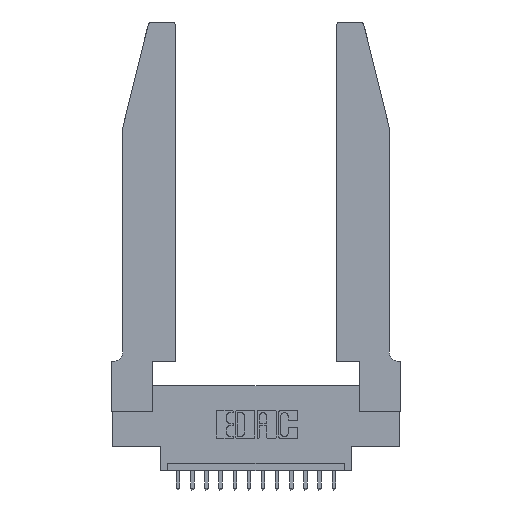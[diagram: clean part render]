
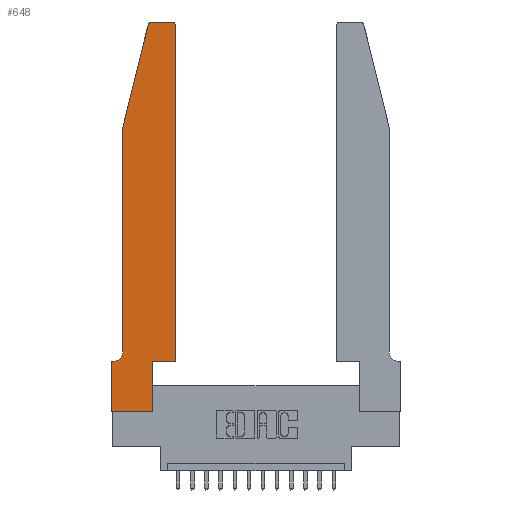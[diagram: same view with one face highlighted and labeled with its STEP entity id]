
A CAD part, top view. The second image highlights one B-rep face of the part: STEP entity #648.
In plain terms, the highlighted planar face has unit normal (0, 0, 1).
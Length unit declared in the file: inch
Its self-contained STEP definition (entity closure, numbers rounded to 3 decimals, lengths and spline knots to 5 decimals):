
#505 = VECTOR ( 'NONE', #3191, 39.37008 ) ;
#648 = ADVANCED_FACE ( 'NONE', ( #2375 ), #1194, .T. ) ;
#860 = CARTESIAN_POINT ( 'NONE',  ( 0.0055, 0.35, 0.37 ) ) ;
#938 = AXIS2_PLACEMENT_3D ( 'NONE', #9740, #6860, #15231 ) ;
#978 = ORIENTED_EDGE ( 'NONE', *, *, #1954, .T. ) ;
#1126 = CARTESIAN_POINT ( 'NONE',  ( 0.4205, 2.72, 0.37 ) ) ;
#1164 = DIRECTION ( 'NONE',  ( 1., 0., 0. ) ) ;
#1194 = PLANE ( 'NONE',  #938 ) ;
#1410 = CIRCLE ( 'NONE', #11759, 0.03 ) ;
#1486 = EDGE_LOOP ( 'NONE', ( #7012, #6989, #10136, #8516, #10337, #12868, #978, #15834, #2929, #10157, #9192, #16131 ) ) ;
#1492 = DIRECTION ( 'NONE',  ( -1., 0., 0. ) ) ;
#1592 = CIRCLE ( 'NONE', #3282, 0.03 ) ;
#1691 = VERTEX_POINT ( 'NONE', #3561 ) ;
#1754 = EDGE_CURVE ( 'NONE', #7570, #12493, #9913, .T. ) ;
#1954 = EDGE_CURVE ( 'NONE', #10175, #7570, #10794, .T. ) ;
#2098 = CARTESIAN_POINT ( 'NONE',  ( 0.2865, 0., 0.37 ) ) ;
#2114 = DIRECTION ( 'NONE',  ( 0., 0., -1. ) ) ;
#2375 = FACE_OUTER_BOUND ( 'NONE', #1486, .T. ) ;
#2431 = VERTEX_POINT ( 'NONE', #11007 ) ;
#2732 = CARTESIAN_POINT ( 'NONE',  ( 0.0755, 0.42, 0.37 ) ) ;
#2853 = CARTESIAN_POINT ( 'NONE',  ( 0.0755, 2., 0.37 ) ) ;
#2929 = ORIENTED_EDGE ( 'NONE', *, *, #4410, .T. ) ;
#3191 = DIRECTION ( 'NONE',  ( -0.239, -0.971, 0. ) ) ;
#3282 = AXIS2_PLACEMENT_3D ( 'NONE', #17812, #9458, #1164 ) ;
#3397 = VECTOR ( 'NONE', #14045, 39.37008 ) ;
#3463 = EDGE_CURVE ( 'NONE', #2431, #10701, #1592, .T. ) ;
#3561 = CARTESIAN_POINT ( 'NONE',  ( 0.4505, 2.72, 0.37 ) ) ;
#3717 = VERTEX_POINT ( 'NONE', #860 ) ;
#3766 = AXIS2_PLACEMENT_3D ( 'NONE', #13324, #2114, #9040 ) ;
#4410 = EDGE_CURVE ( 'NONE', #12493, #5155, #17122, .T. ) ;
#4894 = EDGE_CURVE ( 'NONE', #3717, #10175, #13527, .T. ) ;
#5096 = VECTOR ( 'NONE', #10416, 39.37008 ) ;
#5155 = VERTEX_POINT ( 'NONE', #15409 ) ;
#5196 = EDGE_CURVE ( 'NONE', #10701, #12759, #17670, .T. ) ;
#5198 = VERTEX_POINT ( 'NONE', #5371 ) ;
#5371 = CARTESIAN_POINT ( 'NONE',  ( 0.4505, 0.35, 0.37 ) ) ;
#5412 = CARTESIAN_POINT ( 'NONE',  ( 0.0755, 2., 0.37 ) ) ;
#5843 = CARTESIAN_POINT ( 'NONE',  ( 0.2865, 0.35, 0.37 ) ) ;
#6199 = VECTOR ( 'NONE', #14973, 39.37008 ) ;
#6245 = VECTOR ( 'NONE', #17843, 39.37008 ) ;
#6577 = DIRECTION ( 'NONE',  ( 0., 1., 0. ) ) ;
#6606 = DIRECTION ( 'NONE',  ( 1., 0., 0. ) ) ;
#6827 = EDGE_CURVE ( 'NONE', #5155, #5198, #16113, .T. ) ;
#6860 = DIRECTION ( 'NONE',  ( 0., 0., 1. ) ) ;
#6955 = VECTOR ( 'NONE', #7656, 39.37008 ) ;
#6989 = ORIENTED_EDGE ( 'NONE', *, *, #3463, .T. ) ;
#7012 = ORIENTED_EDGE ( 'NONE', *, *, #11635, .T. ) ;
#7280 = EDGE_CURVE ( 'NONE', #11071, #3717, #8637, .T. ) ;
#7570 = VERTEX_POINT ( 'NONE', #12748 ) ;
#7656 = DIRECTION ( 'NONE',  ( 1., 0., 0. ) ) ;
#8516 = ORIENTED_EDGE ( 'NONE', *, *, #12175, .T. ) ;
#8607 = CARTESIAN_POINT ( 'NONE',  ( 0.4505, 0.35, 0.37 ) ) ;
#8637 = CIRCLE ( 'NONE', #3766, 0.07 ) ;
#8858 = VERTEX_POINT ( 'NONE', #16887 ) ;
#8970 = CARTESIAN_POINT ( 'NONE',  ( 0.4505, 0.35, 0.37 ) ) ;
#9040 = DIRECTION ( 'NONE',  ( -1., 0., 0. ) ) ;
#9192 = ORIENTED_EDGE ( 'NONE', *, *, #15485, .T. ) ;
#9458 = DIRECTION ( 'NONE',  ( 0., 0., 1. ) ) ;
#9634 = LINE ( 'NONE', #2853, #5096 ) ;
#9671 = CARTESIAN_POINT ( 'NONE',  ( 0.0755, 2., 0.37 ) ) ;
#9740 = CARTESIAN_POINT ( 'NONE',  ( 0., 0.35, 0.37 ) ) ;
#9844 = VECTOR ( 'NONE', #1492, 39.37008 ) ;
#9913 = LINE ( 'NONE', #15040, #6245 ) ;
#10136 = ORIENTED_EDGE ( 'NONE', *, *, #5196, .T. ) ;
#10157 = ORIENTED_EDGE ( 'NONE', *, *, #6827, .T. ) ;
#10166 = LINE ( 'NONE', #8607, #15393 ) ;
#10175 = VERTEX_POINT ( 'NONE', #14921 ) ;
#10337 = ORIENTED_EDGE ( 'NONE', *, *, #7280, .T. ) ;
#10416 = DIRECTION ( 'NONE',  ( 0., -1., 0. ) ) ;
#10701 = VERTEX_POINT ( 'NONE', #11785 ) ;
#10794 = LINE ( 'NONE', #16627, #3397 ) ;
#11007 = CARTESIAN_POINT ( 'NONE',  ( 0.284, 2.75, 0.37 ) ) ;
#11071 = VERTEX_POINT ( 'NONE', #2732 ) ;
#11384 = VECTOR ( 'NONE', #6577, 39.37008 ) ;
#11612 = EDGE_CURVE ( 'NONE', #1691, #8858, #1410, .T. ) ;
#11635 = EDGE_CURVE ( 'NONE', #8858, #2431, #12053, .T. ) ;
#11759 = AXIS2_PLACEMENT_3D ( 'NONE', #1126, #17659, #6606 ) ;
#11785 = CARTESIAN_POINT ( 'NONE',  ( 0.25487, 2.72718, 0.37 ) ) ;
#12053 = LINE ( 'NONE', #13506, #6199 ) ;
#12175 = EDGE_CURVE ( 'NONE', #12759, #11071, #9634, .T. ) ;
#12493 = VERTEX_POINT ( 'NONE', #2098 ) ;
#12748 = CARTESIAN_POINT ( 'NONE',  ( 0., 0., 0.37 ) ) ;
#12759 = VERTEX_POINT ( 'NONE', #5412 ) ;
#12868 = ORIENTED_EDGE ( 'NONE', *, *, #4894, .T. ) ;
#13324 = CARTESIAN_POINT ( 'NONE',  ( 0.0055, 0.42, 0.37 ) ) ;
#13506 = CARTESIAN_POINT ( 'NONE',  ( 0.2605, 2.75, 0.37 ) ) ;
#13527 = LINE ( 'NONE', #16750, #9844 ) ;
#14045 = DIRECTION ( 'NONE',  ( 0., -1., 0. ) ) ;
#14921 = CARTESIAN_POINT ( 'NONE',  ( 0., 0.35, 0.37 ) ) ;
#14973 = DIRECTION ( 'NONE',  ( -1., 0., 0. ) ) ;
#15040 = CARTESIAN_POINT ( 'NONE',  ( 0., 0., 0.37 ) ) ;
#15231 = DIRECTION ( 'NONE',  ( 1., 0., 0. ) ) ;
#15393 = VECTOR ( 'NONE', #15577, 39.37008 ) ;
#15409 = CARTESIAN_POINT ( 'NONE',  ( 0.2865, 0.35, 0.37 ) ) ;
#15485 = EDGE_CURVE ( 'NONE', #5198, #1691, #10166, .T. ) ;
#15577 = DIRECTION ( 'NONE',  ( 0., 1., 0. ) ) ;
#15834 = ORIENTED_EDGE ( 'NONE', *, *, #1754, .T. ) ;
#16113 = LINE ( 'NONE', #8970, #6955 ) ;
#16131 = ORIENTED_EDGE ( 'NONE', *, *, #11612, .T. ) ;
#16627 = CARTESIAN_POINT ( 'NONE',  ( 0., 0., 0.37 ) ) ;
#16750 = CARTESIAN_POINT ( 'NONE',  ( 0.0755, 0.35, 0.37 ) ) ;
#16887 = CARTESIAN_POINT ( 'NONE',  ( 0.4205, 2.75, 0.37 ) ) ;
#17122 = LINE ( 'NONE', #5843, #11384 ) ;
#17659 = DIRECTION ( 'NONE',  ( 0., 0., 1. ) ) ;
#17670 = LINE ( 'NONE', #9671, #505 ) ;
#17812 = CARTESIAN_POINT ( 'NONE',  ( 0.284, 2.72, 0.37 ) ) ;
#17843 = DIRECTION ( 'NONE',  ( 1., 0., 0. ) ) ;
